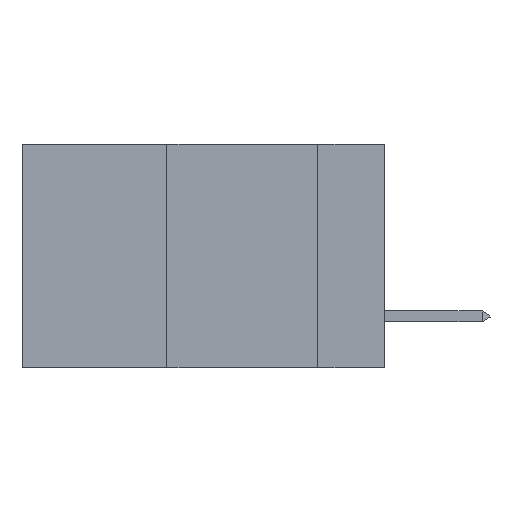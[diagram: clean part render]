
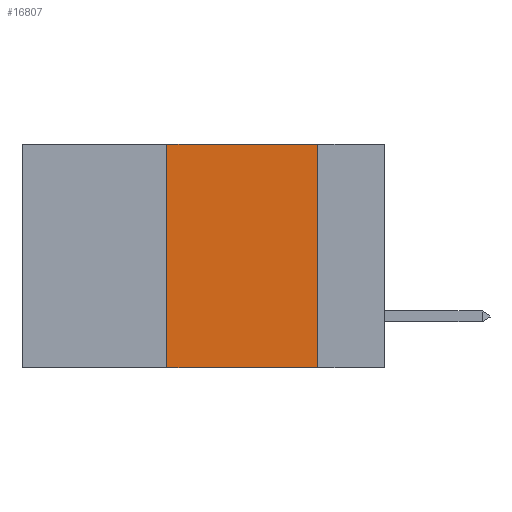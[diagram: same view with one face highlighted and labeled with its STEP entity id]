
A CAD part, left-side view. The second image highlights one B-rep face of the part: STEP entity #16807.
In plain terms, the highlighted planar face has unit normal (-1, 0, 0).
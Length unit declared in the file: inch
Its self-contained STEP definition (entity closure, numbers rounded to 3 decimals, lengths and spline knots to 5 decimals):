
#1676 = LINE ( 'NONE', #8014, #33467 ) ;
#3454 = CARTESIAN_POINT ( 'NONE',  ( 0., 0.6, -0.37 ) ) ;
#5153 = EDGE_CURVE ( 'NONE', #37110, #30003, #20922, .T. ) ;
#5504 = VECTOR ( 'NONE', #25809, 39.37008 ) ;
#5574 = CARTESIAN_POINT ( 'NONE',  ( 0., 0.6, 0. ) ) ;
#6885 = PLANE ( 'NONE',  #43792 ) ;
#8014 = CARTESIAN_POINT ( 'NONE',  ( 0., 0.36, 0. ) ) ;
#8431 = EDGE_CURVE ( 'NONE', #15531, #30003, #39019, .T. ) ;
#11862 = CARTESIAN_POINT ( 'NONE',  ( 0., 0.11, 0. ) ) ;
#13339 = FACE_OUTER_BOUND ( 'NONE', #26792, .T. ) ;
#15531 = VERTEX_POINT ( 'NONE', #11862 ) ;
#16807 = ADVANCED_FACE ( 'NONE', ( #13339 ), #6885, .F. ) ;
#18870 = ORIENTED_EDGE ( 'NONE', *, *, #8431, .F. ) ;
#20520 = VERTEX_POINT ( 'NONE', #35560 ) ;
#20840 = CARTESIAN_POINT ( 'NONE',  ( 0., 0.36, -0.37 ) ) ;
#20922 = LINE ( 'NONE', #3454, #44461 ) ;
#21237 = LINE ( 'NONE', #5574, #44271 ) ;
#22111 = DIRECTION ( 'NONE',  ( 0., 0., -1. ) ) ;
#25809 = DIRECTION ( 'NONE',  ( 0., 0., -1. ) ) ;
#26792 = EDGE_LOOP ( 'NONE', ( #18870, #42798, #37362, #31023 ) ) ;
#29343 = DIRECTION ( 'NONE',  ( 0., -1., 0. ) ) ;
#30003 = VERTEX_POINT ( 'NONE', #34772 ) ;
#31023 = ORIENTED_EDGE ( 'NONE', *, *, #5153, .T. ) ;
#31287 = DIRECTION ( 'NONE',  ( 0., -1., 0. ) ) ;
#33045 = CARTESIAN_POINT ( 'NONE',  ( 0., 0.11, 0. ) ) ;
#33467 = VECTOR ( 'NONE', #37573, 39.37008 ) ;
#34772 = CARTESIAN_POINT ( 'NONE',  ( 0., 0.11, -0.37 ) ) ;
#35560 = CARTESIAN_POINT ( 'NONE',  ( 0., 0.36, 0. ) ) ;
#37110 = VERTEX_POINT ( 'NONE', #20840 ) ;
#37362 = ORIENTED_EDGE ( 'NONE', *, *, #44348, .F. ) ;
#37573 = DIRECTION ( 'NONE',  ( 0., 0., 1. ) ) ;
#39019 = LINE ( 'NONE', #33045, #5504 ) ;
#42798 = ORIENTED_EDGE ( 'NONE', *, *, #46313, .F. ) ;
#43792 = AXIS2_PLACEMENT_3D ( 'NONE', #44131, #44297, #22111 ) ;
#44131 = CARTESIAN_POINT ( 'NONE',  ( 0., 0.6, 0. ) ) ;
#44271 = VECTOR ( 'NONE', #31287, 39.37008 ) ;
#44297 = DIRECTION ( 'NONE',  ( 1., 0., 0. ) ) ;
#44348 = EDGE_CURVE ( 'NONE', #37110, #20520, #1676, .T. ) ;
#44461 = VECTOR ( 'NONE', #29343, 39.37008 ) ;
#46313 = EDGE_CURVE ( 'NONE', #20520, #15531, #21237, .T. ) ;
